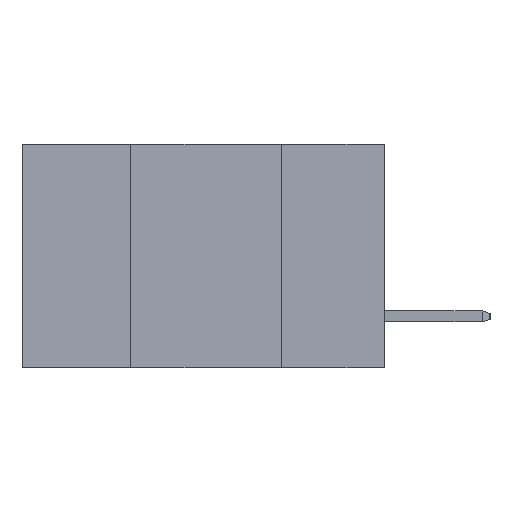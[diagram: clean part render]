
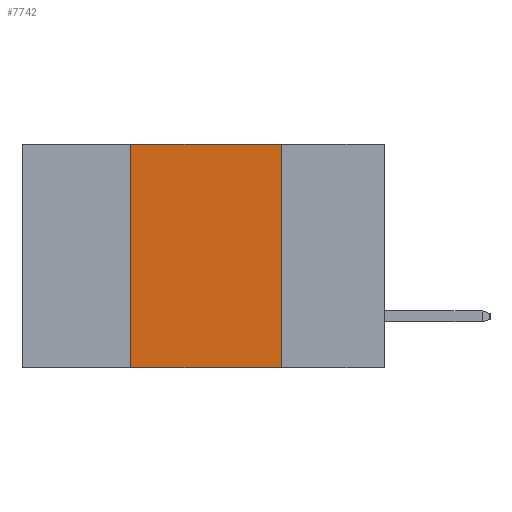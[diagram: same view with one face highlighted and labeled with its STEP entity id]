
A CAD part, left-side view. The second image highlights one B-rep face of the part: STEP entity #7742.
In plain terms, the highlighted planar face has unit normal (-1, 0, 0).
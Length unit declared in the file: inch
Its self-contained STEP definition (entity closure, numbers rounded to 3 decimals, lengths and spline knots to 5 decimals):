
#2169 = VECTOR ( 'NONE', #30703, 39.37008 ) ;
#3443 = FACE_OUTER_BOUND ( 'NONE', #5486, .T. ) ;
#4296 = DIRECTION ( 'NONE',  ( 0., 0., -1. ) ) ;
#5486 = EDGE_LOOP ( 'NONE', ( #6923, #28632, #22616, #8590 ) ) ;
#5799 = CARTESIAN_POINT ( 'NONE',  ( 0., 0.42, 0. ) ) ;
#6237 = CARTESIAN_POINT ( 'NONE',  ( 0., 0.17, -0.37 ) ) ;
#6923 = ORIENTED_EDGE ( 'NONE', *, *, #26883, .F. ) ;
#7742 = ADVANCED_FACE ( 'NONE', ( #3443 ), #10028, .F. ) ;
#8590 = ORIENTED_EDGE ( 'NONE', *, *, #27494, .T. ) ;
#9123 = CARTESIAN_POINT ( 'NONE',  ( 0., 0.42, 0. ) ) ;
#9929 = DIRECTION ( 'NONE',  ( 0., 0., -1. ) ) ;
#9948 = LINE ( 'NONE', #25947, #28390 ) ;
#9994 = DIRECTION ( 'NONE',  ( 1., 0., 0. ) ) ;
#10028 = PLANE ( 'NONE',  #10275 ) ;
#10167 = CARTESIAN_POINT ( 'NONE',  ( 0., 0.6, 0. ) ) ;
#10275 = AXIS2_PLACEMENT_3D ( 'NONE', #10167, #9994, #9929 ) ;
#11040 = LINE ( 'NONE', #30696, #30263 ) ;
#12442 = EDGE_CURVE ( 'NONE', #24228, #29687, #19492, .T. ) ;
#13088 = VECTOR ( 'NONE', #14037, 39.37008 ) ;
#13932 = CARTESIAN_POINT ( 'NONE',  ( 0., 0.17, 0. ) ) ;
#14037 = DIRECTION ( 'NONE',  ( 0., 0., 1. ) ) ;
#14779 = VERTEX_POINT ( 'NONE', #6237 ) ;
#16307 = DIRECTION ( 'NONE',  ( 0., -1., 0. ) ) ;
#18702 = CARTESIAN_POINT ( 'NONE',  ( 0., 0.6, 0. ) ) ;
#19492 = LINE ( 'NONE', #9123, #13088 ) ;
#22382 = EDGE_CURVE ( 'NONE', #29687, #28808, #27936, .T. ) ;
#22616 = ORIENTED_EDGE ( 'NONE', *, *, #12442, .F. ) ;
#24228 = VERTEX_POINT ( 'NONE', #28388 ) ;
#25947 = CARTESIAN_POINT ( 'NONE',  ( 0., 0.17, 0. ) ) ;
#26883 = EDGE_CURVE ( 'NONE', #28808, #14779, #9948, .T. ) ;
#27494 = EDGE_CURVE ( 'NONE', #24228, #14779, #11040, .T. ) ;
#27936 = LINE ( 'NONE', #18702, #2169 ) ;
#28388 = CARTESIAN_POINT ( 'NONE',  ( 0., 0.42, -0.37 ) ) ;
#28390 = VECTOR ( 'NONE', #4296, 39.37008 ) ;
#28632 = ORIENTED_EDGE ( 'NONE', *, *, #22382, .F. ) ;
#28808 = VERTEX_POINT ( 'NONE', #13932 ) ;
#29687 = VERTEX_POINT ( 'NONE', #5799 ) ;
#30263 = VECTOR ( 'NONE', #16307, 39.37008 ) ;
#30696 = CARTESIAN_POINT ( 'NONE',  ( 0., 0.6, -0.37 ) ) ;
#30703 = DIRECTION ( 'NONE',  ( 0., -1., 0. ) ) ;
